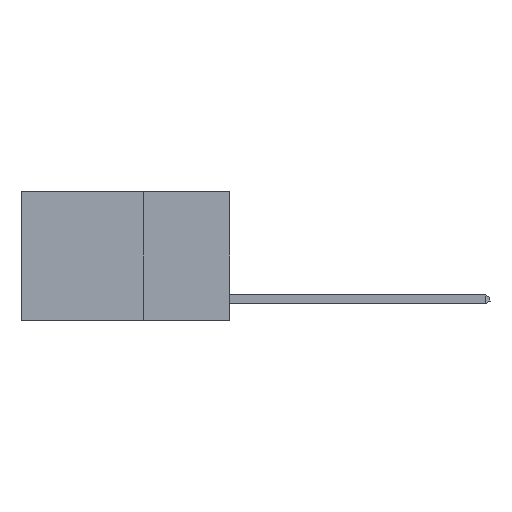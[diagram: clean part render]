
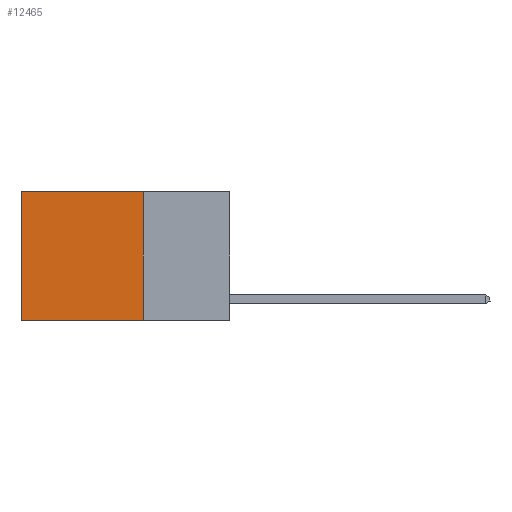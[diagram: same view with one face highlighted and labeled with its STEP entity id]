
A CAD part, left-side view. The second image highlights one B-rep face of the part: STEP entity #12465.
In plain terms, the highlighted planar face has unit normal (-1, 0, 0).
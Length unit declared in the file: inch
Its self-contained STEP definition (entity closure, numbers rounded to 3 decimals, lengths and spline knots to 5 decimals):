
#36 = EDGE_CURVE ( 'NONE', #6414, #4056, #7405, .T. ) ;
#433 = DIRECTION ( 'NONE',  ( 0., 0., -1. ) ) ;
#1051 = CARTESIAN_POINT ( 'NONE',  ( 0.2625, 0.25, 0. ) ) ;
#2549 = CARTESIAN_POINT ( 'NONE',  ( 0.2625, 0.25, 0. ) ) ;
#2763 = EDGE_CURVE ( 'NONE', #7219, #6414, #16871, .T. ) ;
#3222 = ORIENTED_EDGE ( 'NONE', *, *, #8264, .T. ) ;
#3251 = VERTEX_POINT ( 'NONE', #9962 ) ;
#3503 = LINE ( 'NONE', #2549, #13043 ) ;
#3716 = ORIENTED_EDGE ( 'NONE', *, *, #2763, .F. ) ;
#4056 = VERTEX_POINT ( 'NONE', #5597 ) ;
#4108 = CARTESIAN_POINT ( 'NONE',  ( 0.2625, 0.25, 0. ) ) ;
#4668 = ORIENTED_EDGE ( 'NONE', *, *, #6639, .T. ) ;
#5597 = CARTESIAN_POINT ( 'NONE',  ( 0.2625, 0.6, -0.37 ) ) ;
#5791 = VECTOR ( 'NONE', #12311, 39.37008 ) ;
#6032 = DIRECTION ( 'NONE',  ( 0., 0., -1. ) ) ;
#6414 = VERTEX_POINT ( 'NONE', #9264 ) ;
#6639 = EDGE_CURVE ( 'NONE', #3251, #4056, #11166, .T. ) ;
#7219 = VERTEX_POINT ( 'NONE', #4108 ) ;
#7405 = LINE ( 'NONE', #8691, #10849 ) ;
#8264 = EDGE_CURVE ( 'NONE', #7219, #3251, #3503, .T. ) ;
#8691 = CARTESIAN_POINT ( 'NONE',  ( 0.2625, 0.25, -0.37 ) ) ;
#9002 = PLANE ( 'NONE',  #11755 ) ;
#9264 = CARTESIAN_POINT ( 'NONE',  ( 0.2625, 0.25, -0.37 ) ) ;
#9962 = CARTESIAN_POINT ( 'NONE',  ( 0.2625, 0.6, 0. ) ) ;
#10202 = DIRECTION ( 'NONE',  ( 1., 0., 0. ) ) ;
#10235 = DIRECTION ( 'NONE',  ( 0., 1., 0. ) ) ;
#10545 = ORIENTED_EDGE ( 'NONE', *, *, #36, .F. ) ;
#10716 = VECTOR ( 'NONE', #433, 39.37008 ) ;
#10849 = VECTOR ( 'NONE', #10235, 39.37008 ) ;
#11166 = LINE ( 'NONE', #14471, #10716 ) ;
#11755 = AXIS2_PLACEMENT_3D ( 'NONE', #17122, #10202, #6032 ) ;
#11794 = FACE_OUTER_BOUND ( 'NONE', #16700, .T. ) ;
#12255 = DIRECTION ( 'NONE',  ( 0., 1., 0. ) ) ;
#12311 = DIRECTION ( 'NONE',  ( 0., 0., -1. ) ) ;
#12465 = ADVANCED_FACE ( 'NONE', ( #11794 ), #9002, .F. ) ;
#13043 = VECTOR ( 'NONE', #12255, 39.37008 ) ;
#14471 = CARTESIAN_POINT ( 'NONE',  ( 0.2625, 0.6, 0. ) ) ;
#16700 = EDGE_LOOP ( 'NONE', ( #4668, #10545, #3716, #3222 ) ) ;
#16871 = LINE ( 'NONE', #1051, #5791 ) ;
#17122 = CARTESIAN_POINT ( 'NONE',  ( 0.2625, 0.25, 0. ) ) ;
